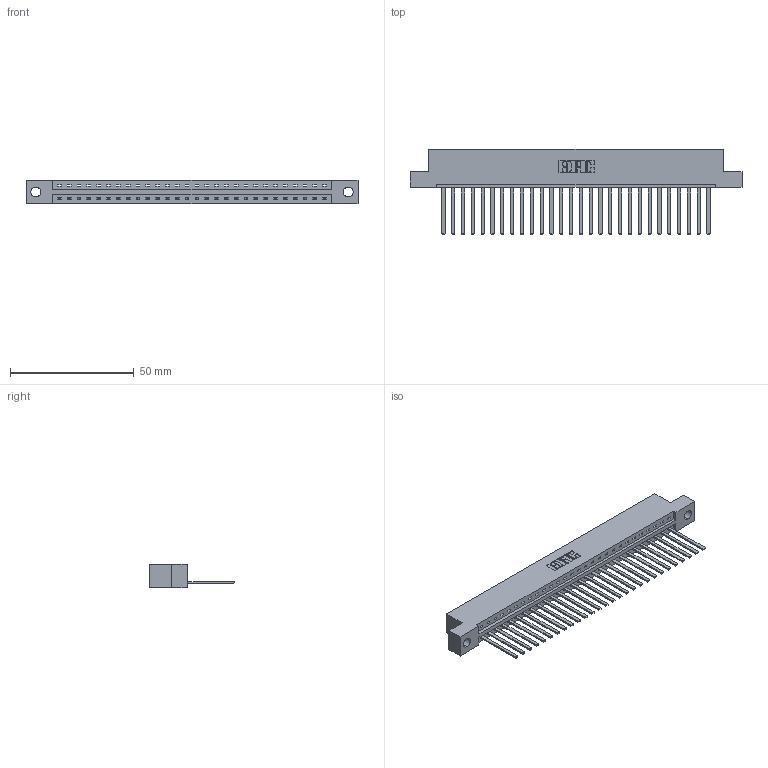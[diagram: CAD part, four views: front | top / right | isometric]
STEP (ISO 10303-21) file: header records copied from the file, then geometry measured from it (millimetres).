
FILE_DESCRIPTION (( 'STEP AP203' ), '1' );
FILE_NAME ('337-028-544-104.STEP', '2019-09-30T21:24:36', ( '' ), ( '' ), 'SwSTEP 2.0', 'SolidWorks 2016', '' );
FILE_SCHEMA (( 'CONFIG_CONTROL_DESIGN' ));
Length unit declared in the file: inch
Products named in the file (3): 345-292-001_345-293-144; 337 Part_Flush Mounting Lugs - 0.156 Dia-TH; 337-028-544-104
Assembly tree (29 placements, depth 2):
  337-028-544-104
    337 Part_Flush Mounting Lugs - 0.156 Dia-TH
    345-292-001_345-293-144  x28
Bounding box: 133.96 x 34.3 x 9.4 mm (x, y, z)
Volume: 13984.1 mm3; surface area: 15234.8 mm2
Topology: 29 solids, 29 shells, 1682 faces, 5071 edges, 3342 vertices
Faces by surface type: plane 1246, cylinder 436
Entity records: 22443 total; most frequent: CARTESIAN_POINT 3914, ORIENTED_EDGE 3878, DIRECTION 3319, EDGE_CURVE 1939, VECTOR 1815, LINE 1815, VERTEX_POINT 1290, AXIS2_PLACEMENT_3D 752
